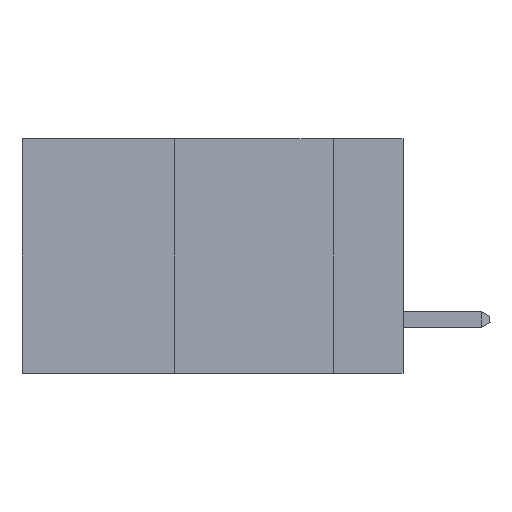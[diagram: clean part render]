
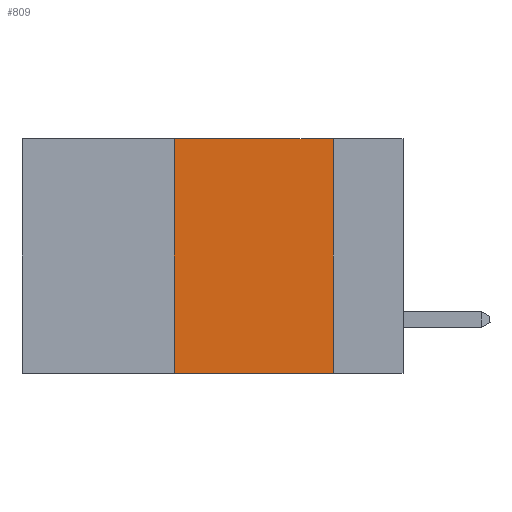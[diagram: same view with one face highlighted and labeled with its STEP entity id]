
A CAD part, left-side view. The second image highlights one B-rep face of the part: STEP entity #809.
In plain terms, the highlighted planar face has unit normal (-1, 0, 0).
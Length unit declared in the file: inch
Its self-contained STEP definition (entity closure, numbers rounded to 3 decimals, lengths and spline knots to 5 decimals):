
#729 = DIRECTION ( 'NONE',  ( 1., 0., 0. ) ) ;
#809 = ADVANCED_FACE ( 'NONE', ( #2655 ), #6041, .F. ) ;
#985 = CARTESIAN_POINT ( 'NONE',  ( 0., 0.6, 0. ) ) ;
#994 = ORIENTED_EDGE ( 'NONE', *, *, #11564, .T. ) ;
#1063 = LINE ( 'NONE', #14258, #7342 ) ;
#1318 = CARTESIAN_POINT ( 'NONE',  ( 0., 0.11, -0.37 ) ) ;
#1641 = DIRECTION ( 'NONE',  ( 0., 0., -1. ) ) ;
#2413 = LINE ( 'NONE', #9223, #14242 ) ;
#2582 = VERTEX_POINT ( 'NONE', #1318 ) ;
#2615 = LINE ( 'NONE', #985, #10696 ) ;
#2655 = FACE_OUTER_BOUND ( 'NONE', #12269, .T. ) ;
#2833 = VECTOR ( 'NONE', #15759, 39.37008 ) ;
#4363 = CARTESIAN_POINT ( 'NONE',  ( 0., 0.6, 0. ) ) ;
#5783 = ORIENTED_EDGE ( 'NONE', *, *, #12322, .F. ) ;
#6041 = PLANE ( 'NONE',  #7955 ) ;
#7342 = VECTOR ( 'NONE', #1641, 39.37008 ) ;
#7955 = AXIS2_PLACEMENT_3D ( 'NONE', #4363, #729, #13138 ) ;
#8034 = CARTESIAN_POINT ( 'NONE',  ( 0., 0.36, -0.37 ) ) ;
#8126 = DIRECTION ( 'NONE',  ( 0., 0., 1. ) ) ;
#9223 = CARTESIAN_POINT ( 'NONE',  ( 0., 0.36, 0. ) ) ;
#9343 = VERTEX_POINT ( 'NONE', #10613 ) ;
#9525 = LINE ( 'NONE', #11874, #2833 ) ;
#10613 = CARTESIAN_POINT ( 'NONE',  ( 0., 0.11, 0. ) ) ;
#10696 = VECTOR ( 'NONE', #14985, 39.37008 ) ;
#10979 = ORIENTED_EDGE ( 'NONE', *, *, #12897, .F. ) ;
#11564 = EDGE_CURVE ( 'NONE', #13935, #2582, #9525, .T. ) ;
#11874 = CARTESIAN_POINT ( 'NONE',  ( 0., 0.6, -0.37 ) ) ;
#11902 = VERTEX_POINT ( 'NONE', #13797 ) ;
#12075 = ORIENTED_EDGE ( 'NONE', *, *, #14790, .F. ) ;
#12269 = EDGE_LOOP ( 'NONE', ( #10979, #5783, #12075, #994 ) ) ;
#12322 = EDGE_CURVE ( 'NONE', #11902, #9343, #2615, .T. ) ;
#12897 = EDGE_CURVE ( 'NONE', #9343, #2582, #1063, .T. ) ;
#13138 = DIRECTION ( 'NONE',  ( 0., 0., -1. ) ) ;
#13797 = CARTESIAN_POINT ( 'NONE',  ( 0., 0.36, 0. ) ) ;
#13935 = VERTEX_POINT ( 'NONE', #8034 ) ;
#14242 = VECTOR ( 'NONE', #8126, 39.37008 ) ;
#14258 = CARTESIAN_POINT ( 'NONE',  ( 0., 0.11, 0. ) ) ;
#14790 = EDGE_CURVE ( 'NONE', #13935, #11902, #2413, .T. ) ;
#14985 = DIRECTION ( 'NONE',  ( 0., -1., 0. ) ) ;
#15759 = DIRECTION ( 'NONE',  ( 0., -1., 0. ) ) ;
